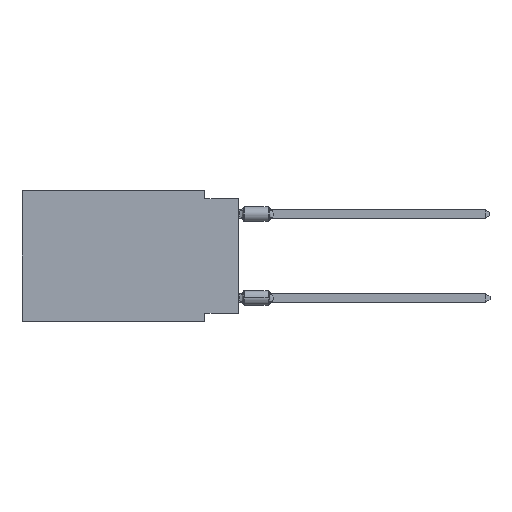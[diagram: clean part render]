
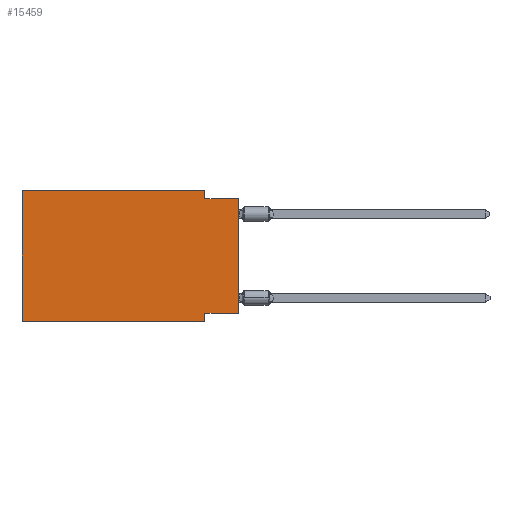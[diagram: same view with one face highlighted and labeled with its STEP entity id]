
A CAD part, left-side view. The second image highlights one B-rep face of the part: STEP entity #15459.
In plain terms, the highlighted planar face has unit normal (-1, 0, 0).
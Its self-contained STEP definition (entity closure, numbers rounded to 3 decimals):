
#320 = PLANE ( 'NONE',  #2531 ) ;
#653 = ORIENTED_EDGE ( 'NONE', *, *, #5214, .F. ) ;
#954 = CARTESIAN_POINT ( 'NONE',  ( 0., 2.54, -9.906 ) ) ;
#1031 = EDGE_CURVE ( 'NONE', #21176, #20899, #18047, .T. ) ;
#1267 = CARTESIAN_POINT ( 'NONE',  ( 0., 2.54, -9.271 ) ) ;
#1587 = CARTESIAN_POINT ( 'NONE',  ( 0., 16.383, 0. ) ) ;
#1631 = VECTOR ( 'NONE', #6112, 1000. ) ;
#1999 = VECTOR ( 'NONE', #16586, 1000. ) ;
#2147 = CARTESIAN_POINT ( 'NONE',  ( 0., 0., 0. ) ) ;
#2185 = DIRECTION ( 'NONE',  ( 0., 1., 0. ) ) ;
#2424 = VECTOR ( 'NONE', #10440, 1000. ) ;
#2531 = AXIS2_PLACEMENT_3D ( 'NONE', #15642, #10368, #21062 ) ;
#3190 = CARTESIAN_POINT ( 'NONE',  ( 0., 16.383, -9.906 ) ) ;
#3537 = DIRECTION ( 'NONE',  ( 0., -1., 0. ) ) ;
#4043 = VECTOR ( 'NONE', #3537, 1000. ) ;
#4718 = LINE ( 'NONE', #6447, #1631 ) ;
#4837 = CARTESIAN_POINT ( 'NONE',  ( 0., 0., -9.271 ) ) ;
#5214 = EDGE_CURVE ( 'NONE', #8519, #10962, #9914, .T. ) ;
#5398 = VERTEX_POINT ( 'NONE', #19573 ) ;
#6112 = DIRECTION ( 'NONE',  ( 0., -1., 0. ) ) ;
#6447 = CARTESIAN_POINT ( 'NONE',  ( 0., 0., -0.635 ) ) ;
#6517 = LINE ( 'NONE', #10333, #2424 ) ;
#7586 = ORIENTED_EDGE ( 'NONE', *, *, #19614, .F. ) ;
#7933 = ORIENTED_EDGE ( 'NONE', *, *, #21554, .F. ) ;
#8064 = EDGE_CURVE ( 'NONE', #11320, #21176, #13689, .T. ) ;
#8169 = CARTESIAN_POINT ( 'NONE',  ( 0., 2.54, -0.635 ) ) ;
#8185 = CARTESIAN_POINT ( 'NONE',  ( 0., 2.54, -9.906 ) ) ;
#8519 = VERTEX_POINT ( 'NONE', #1267 ) ;
#8573 = EDGE_CURVE ( 'NONE', #12768, #5398, #4718, .T. ) ;
#8696 = VERTEX_POINT ( 'NONE', #4837 ) ;
#8971 = FACE_OUTER_BOUND ( 'NONE', #11528, .T. ) ;
#9525 = CARTESIAN_POINT ( 'NONE',  ( 0., 16.383, 0. ) ) ;
#9914 = LINE ( 'NONE', #8185, #1999 ) ;
#10279 = EDGE_CURVE ( 'NONE', #11320, #10962, #15522, .T. ) ;
#10333 = CARTESIAN_POINT ( 'NONE',  ( 0., 2.54, 0. ) ) ;
#10368 = DIRECTION ( 'NONE',  ( 1., 0., 0. ) ) ;
#10440 = DIRECTION ( 'NONE',  ( 0., 0., -1. ) ) ;
#10695 = CARTESIAN_POINT ( 'NONE',  ( 0., 16.383, 0. ) ) ;
#10891 = VECTOR ( 'NONE', #2185, 1000. ) ;
#10912 = DIRECTION ( 'NONE',  ( 0., 0., 1. ) ) ;
#10962 = VERTEX_POINT ( 'NONE', #954 ) ;
#11320 = VERTEX_POINT ( 'NONE', #18556 ) ;
#11368 = DIRECTION ( 'NONE',  ( 0., -1., 0. ) ) ;
#11528 = EDGE_LOOP ( 'NONE', ( #21200, #13246, #7933, #21889, #18364, #15875, #653, #7586 ) ) ;
#11593 = LINE ( 'NONE', #21417, #10891 ) ;
#12768 = VERTEX_POINT ( 'NONE', #8169 ) ;
#13246 = ORIENTED_EDGE ( 'NONE', *, *, #8573, .F. ) ;
#13689 = LINE ( 'NONE', #1587, #14127 ) ;
#14127 = VECTOR ( 'NONE', #15523, 1000. ) ;
#14913 = VECTOR ( 'NONE', #11368, 1000. ) ;
#15459 = ADVANCED_FACE ( 'NONE', ( #8971 ), #320, .F. ) ;
#15522 = LINE ( 'NONE', #3190, #4043 ) ;
#15523 = DIRECTION ( 'NONE',  ( 0., 0., 1. ) ) ;
#15642 = CARTESIAN_POINT ( 'NONE',  ( 0., 16.383, 0. ) ) ;
#15875 = ORIENTED_EDGE ( 'NONE', *, *, #10279, .T. ) ;
#16586 = DIRECTION ( 'NONE',  ( 0., 0., -1. ) ) ;
#18047 = LINE ( 'NONE', #9525, #14913 ) ;
#18259 = EDGE_CURVE ( 'NONE', #8696, #5398, #21491, .T. ) ;
#18364 = ORIENTED_EDGE ( 'NONE', *, *, #8064, .F. ) ;
#18556 = CARTESIAN_POINT ( 'NONE',  ( 0., 16.383, -9.906 ) ) ;
#19573 = CARTESIAN_POINT ( 'NONE',  ( 0., 0., -0.635 ) ) ;
#19614 = EDGE_CURVE ( 'NONE', #8696, #8519, #11593, .T. ) ;
#20645 = VECTOR ( 'NONE', #10912, 1000. ) ;
#20899 = VERTEX_POINT ( 'NONE', #22104 ) ;
#21062 = DIRECTION ( 'NONE',  ( 0., 0., -1. ) ) ;
#21176 = VERTEX_POINT ( 'NONE', #10695 ) ;
#21200 = ORIENTED_EDGE ( 'NONE', *, *, #18259, .T. ) ;
#21417 = CARTESIAN_POINT ( 'NONE',  ( 0., 0., -9.271 ) ) ;
#21491 = LINE ( 'NONE', #2147, #20645 ) ;
#21554 = EDGE_CURVE ( 'NONE', #20899, #12768, #6517, .T. ) ;
#21889 = ORIENTED_EDGE ( 'NONE', *, *, #1031, .F. ) ;
#22104 = CARTESIAN_POINT ( 'NONE',  ( 0., 2.54, 0. ) ) ;
